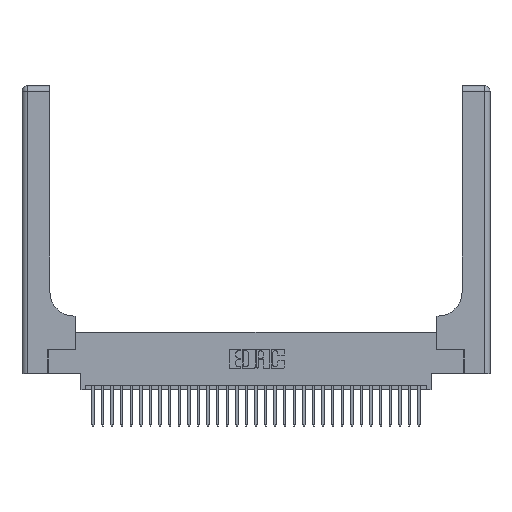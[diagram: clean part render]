
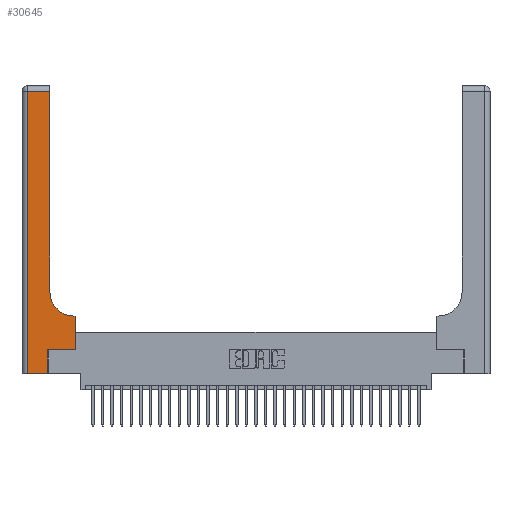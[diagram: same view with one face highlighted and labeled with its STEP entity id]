
A CAD part, top view. The second image highlights one B-rep face of the part: STEP entity #30645.
In plain terms, the highlighted planar face has unit normal (0, 0, 1).
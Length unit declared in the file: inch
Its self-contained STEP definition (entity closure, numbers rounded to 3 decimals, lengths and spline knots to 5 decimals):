
#84 = ORIENTED_EDGE ( 'NONE', *, *, #23971, .T. ) ;
#151 = CARTESIAN_POINT ( 'NONE',  ( 0.06, 0., 0.37 ) ) ;
#823 = ORIENTED_EDGE ( 'NONE', *, *, #4692, .T. ) ;
#1016 = EDGE_LOOP ( 'NONE', ( #25834, #16628, #27780, #84, #9929, #823, #25225, #5817, #21984 ) ) ;
#1603 = DIRECTION ( 'NONE',  ( 1., 0., 0. ) ) ;
#2221 = DIRECTION ( 'NONE',  ( 0., 1., 0. ) ) ;
#2818 = EDGE_CURVE ( 'NONE', #32209, #11141, #14632, .T. ) ;
#3299 = CARTESIAN_POINT ( 'NONE',  ( 0.5585, 0.25, 0.37 ) ) ;
#3825 = CARTESIAN_POINT ( 'NONE',  ( 0., 3., 0.37 ) ) ;
#3882 = FACE_OUTER_BOUND ( 'NONE', #1016, .T. ) ;
#4692 = EDGE_CURVE ( 'NONE', #9540, #31864, #8753, .T. ) ;
#5072 = CARTESIAN_POINT ( 'NONE',  ( 0.269, 0., 0.37 ) ) ;
#5140 = EDGE_CURVE ( 'NONE', #12122, #11850, #9529, .T. ) ;
#5327 = CARTESIAN_POINT ( 'NONE',  ( 0.5585, 0.25, 0.37 ) ) ;
#5340 = LINE ( 'NONE', #22864, #32258 ) ;
#5343 = EDGE_CURVE ( 'NONE', #6115, #32209, #7894, .T. ) ;
#5406 = VERTEX_POINT ( 'NONE', #19722 ) ;
#5441 = DIRECTION ( 'NONE',  ( 0., 1., 0. ) ) ;
#5817 = ORIENTED_EDGE ( 'NONE', *, *, #15462, .T. ) ;
#6115 = VERTEX_POINT ( 'NONE', #13401 ) ;
#6541 = PLANE ( 'NONE',  #9269 ) ;
#7472 = LINE ( 'NONE', #20036, #18905 ) ;
#7894 = CIRCLE ( 'NONE', #10583, 0.25 ) ;
#8753 = LINE ( 'NONE', #24054, #26737 ) ;
#9036 = VECTOR ( 'NONE', #24299, 39.37008 ) ;
#9269 = AXIS2_PLACEMENT_3D ( 'NONE', #3825, #16945, #17061 ) ;
#9529 = LINE ( 'NONE', #31352, #9952 ) ;
#9540 = VERTEX_POINT ( 'NONE', #12135 ) ;
#9712 = VECTOR ( 'NONE', #2221, 39.37008 ) ;
#9929 = ORIENTED_EDGE ( 'NONE', *, *, #30386, .T. ) ;
#9952 = VECTOR ( 'NONE', #31975, 39.37008 ) ;
#10209 = CARTESIAN_POINT ( 'NONE',  ( 0.2915, 0.85, 0.37 ) ) ;
#10445 = DIRECTION ( 'NONE',  ( 0., 1., 0. ) ) ;
#10583 = AXIS2_PLACEMENT_3D ( 'NONE', #27600, #27819, #1603 ) ;
#11141 = VERTEX_POINT ( 'NONE', #16808 ) ;
#11850 = VERTEX_POINT ( 'NONE', #151 ) ;
#12122 = VERTEX_POINT ( 'NONE', #22918 ) ;
#12135 = CARTESIAN_POINT ( 'NONE',  ( 0.269, 0.25, 0.37 ) ) ;
#12476 = EDGE_CURVE ( 'NONE', #11141, #12122, #12715, .T. ) ;
#12715 = LINE ( 'NONE', #24645, #9036 ) ;
#12874 = VECTOR ( 'NONE', #10445, 39.37008 ) ;
#13401 = CARTESIAN_POINT ( 'NONE',  ( 0.5415, 0.6, 0.37 ) ) ;
#14322 = EDGE_CURVE ( 'NONE', #31864, #31524, #32593, .T. ) ;
#14632 = LINE ( 'NONE', #22865, #9712 ) ;
#14706 = DIRECTION ( 'NONE',  ( 1., 0., 0. ) ) ;
#15462 = EDGE_CURVE ( 'NONE', #31524, #6115, #5340, .T. ) ;
#16294 = DIRECTION ( 'NONE',  ( 1., 0., 0. ) ) ;
#16628 = ORIENTED_EDGE ( 'NONE', *, *, #12476, .T. ) ;
#16808 = CARTESIAN_POINT ( 'NONE',  ( 0.2915, 2.94, 0.37 ) ) ;
#16945 = DIRECTION ( 'NONE',  ( 0., 0., -1. ) ) ;
#17061 = DIRECTION ( 'NONE',  ( -1., 0., 0. ) ) ;
#18905 = VECTOR ( 'NONE', #14706, 39.37008 ) ;
#19722 = CARTESIAN_POINT ( 'NONE',  ( 0.269, 0., 0.37 ) ) ;
#20036 = CARTESIAN_POINT ( 'NONE',  ( 0., 0., 0.37 ) ) ;
#20608 = LINE ( 'NONE', #5072, #12874 ) ;
#21984 = ORIENTED_EDGE ( 'NONE', *, *, #5343, .T. ) ;
#22864 = CARTESIAN_POINT ( 'NONE',  ( 0.2915, 0.6, 0.37 ) ) ;
#22865 = CARTESIAN_POINT ( 'NONE',  ( 0.2915, 3., 0.37 ) ) ;
#22918 = CARTESIAN_POINT ( 'NONE',  ( 0.06, 2.94, 0.37 ) ) ;
#23971 = EDGE_CURVE ( 'NONE', #11850, #5406, #7472, .T. ) ;
#24024 = VECTOR ( 'NONE', #5441, 39.37008 ) ;
#24054 = CARTESIAN_POINT ( 'NONE',  ( 0.269, 0.25, 0.37 ) ) ;
#24299 = DIRECTION ( 'NONE',  ( -1., 0., 0. ) ) ;
#24645 = CARTESIAN_POINT ( 'NONE',  ( 0., 2.94, 0.37 ) ) ;
#25225 = ORIENTED_EDGE ( 'NONE', *, *, #14322, .T. ) ;
#25710 = DIRECTION ( 'NONE',  ( -1., 0., 0. ) ) ;
#25834 = ORIENTED_EDGE ( 'NONE', *, *, #2818, .T. ) ;
#26737 = VECTOR ( 'NONE', #16294, 39.37008 ) ;
#27600 = CARTESIAN_POINT ( 'NONE',  ( 0.5415, 0.85, 0.37 ) ) ;
#27780 = ORIENTED_EDGE ( 'NONE', *, *, #5140, .T. ) ;
#27819 = DIRECTION ( 'NONE',  ( 0., 0., -1. ) ) ;
#30386 = EDGE_CURVE ( 'NONE', #5406, #9540, #20608, .T. ) ;
#30645 = ADVANCED_FACE ( 'NONE', ( #3882 ), #6541, .F. ) ;
#31042 = CARTESIAN_POINT ( 'NONE',  ( 0.5585, 0.6, 0.37 ) ) ;
#31352 = CARTESIAN_POINT ( 'NONE',  ( 0.06, 3., 0.37 ) ) ;
#31524 = VERTEX_POINT ( 'NONE', #31042 ) ;
#31864 = VERTEX_POINT ( 'NONE', #3299 ) ;
#31975 = DIRECTION ( 'NONE',  ( 0., -1., 0. ) ) ;
#32209 = VERTEX_POINT ( 'NONE', #10209 ) ;
#32258 = VECTOR ( 'NONE', #25710, 39.37008 ) ;
#32593 = LINE ( 'NONE', #5327, #24024 ) ;
